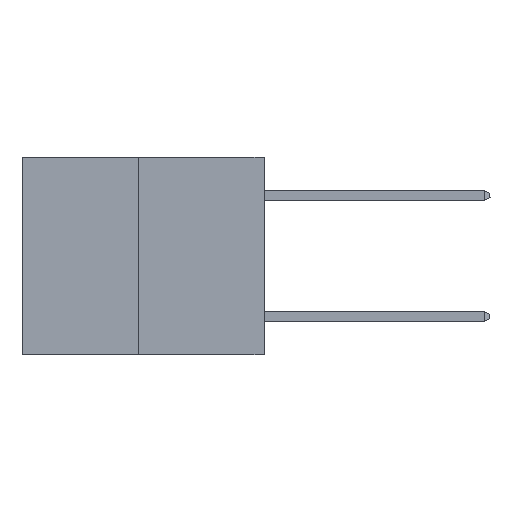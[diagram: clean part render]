
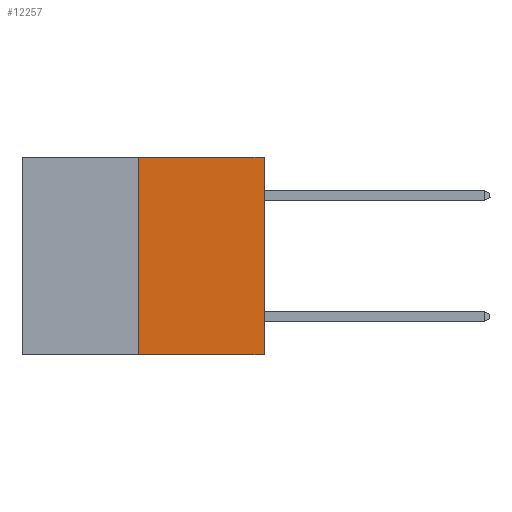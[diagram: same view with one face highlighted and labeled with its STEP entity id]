
A CAD part, left-side view. The second image highlights one B-rep face of the part: STEP entity #12257.
In plain terms, the highlighted planar face has unit normal (-1, 0, 0).
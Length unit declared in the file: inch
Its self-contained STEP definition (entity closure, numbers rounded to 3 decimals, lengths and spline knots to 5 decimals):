
#438 = DIRECTION ( 'NONE',  ( 0., -1., 0. ) ) ;
#1742 = LINE ( 'NONE', #10830, #18817 ) ;
#2814 = LINE ( 'NONE', #4775, #24512 ) ;
#3257 = VERTEX_POINT ( 'NONE', #18724 ) ;
#4295 = VERTEX_POINT ( 'NONE', #26055 ) ;
#4759 = EDGE_LOOP ( 'NONE', ( #13429, #23519, #9899, #19795 ) ) ;
#4775 = CARTESIAN_POINT ( 'NONE',  ( 0., 0., 0. ) ) ;
#7463 = DIRECTION ( 'NONE',  ( 0., -1., 0. ) ) ;
#7623 = CARTESIAN_POINT ( 'NONE',  ( 0., 0.312, -0.49 ) ) ;
#7834 = LINE ( 'NONE', #7623, #9478 ) ;
#8848 = FACE_OUTER_BOUND ( 'NONE', #4759, .T. ) ;
#8859 = CARTESIAN_POINT ( 'NONE',  ( 0., 0.6, 0. ) ) ;
#9478 = VECTOR ( 'NONE', #24604, 39.37008 ) ;
#9568 = CARTESIAN_POINT ( 'NONE',  ( 0., 0.6, 0. ) ) ;
#9899 = ORIENTED_EDGE ( 'NONE', *, *, #14182, .T. ) ;
#10830 = CARTESIAN_POINT ( 'NONE',  ( 0., 0.6, -0.49 ) ) ;
#12257 = ADVANCED_FACE ( 'NONE', ( #8848 ), #21421, .F. ) ;
#12821 = EDGE_CURVE ( 'NONE', #18693, #15986, #7834, .T. ) ;
#13429 = ORIENTED_EDGE ( 'NONE', *, *, #12821, .F. ) ;
#14182 = EDGE_CURVE ( 'NONE', #4295, #3257, #2814, .T. ) ;
#15705 = EDGE_CURVE ( 'NONE', #15986, #3257, #16874, .T. ) ;
#15986 = VERTEX_POINT ( 'NONE', #20310 ) ;
#16874 = LINE ( 'NONE', #9568, #21782 ) ;
#18693 = VERTEX_POINT ( 'NONE', #25809 ) ;
#18724 = CARTESIAN_POINT ( 'NONE',  ( 0., 0., 0. ) ) ;
#18817 = VECTOR ( 'NONE', #438, 39.37008 ) ;
#19795 = ORIENTED_EDGE ( 'NONE', *, *, #15705, .F. ) ;
#19965 = EDGE_CURVE ( 'NONE', #18693, #4295, #1742, .T. ) ;
#20310 = CARTESIAN_POINT ( 'NONE',  ( 0., 0.312, 0. ) ) ;
#21421 = PLANE ( 'NONE',  #26489 ) ;
#21782 = VECTOR ( 'NONE', #7463, 39.37008 ) ;
#23519 = ORIENTED_EDGE ( 'NONE', *, *, #19965, .T. ) ;
#23552 = DIRECTION ( 'NONE',  ( 1., 0., 0. ) ) ;
#23899 = DIRECTION ( 'NONE',  ( 0., 0., 1. ) ) ;
#24512 = VECTOR ( 'NONE', #23899, 39.37008 ) ;
#24604 = DIRECTION ( 'NONE',  ( 0., 0., 1. ) ) ;
#25685 = DIRECTION ( 'NONE',  ( 0., 0., -1. ) ) ;
#25809 = CARTESIAN_POINT ( 'NONE',  ( 0., 0.312, -0.49 ) ) ;
#26055 = CARTESIAN_POINT ( 'NONE',  ( 0., 0., -0.49 ) ) ;
#26489 = AXIS2_PLACEMENT_3D ( 'NONE', #8859, #23552, #25685 ) ;
